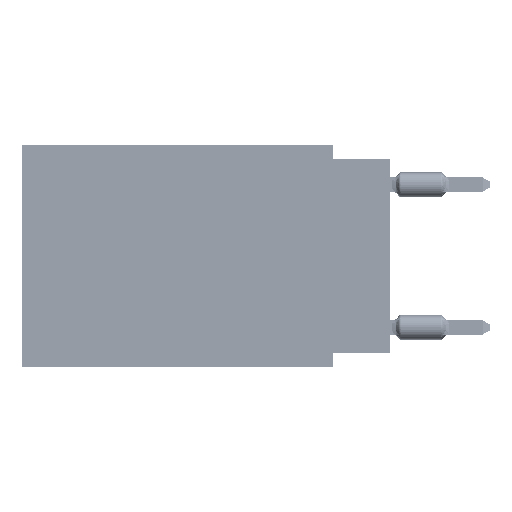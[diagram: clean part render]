
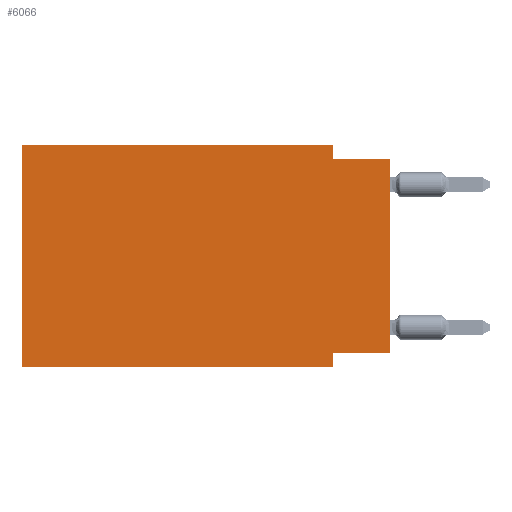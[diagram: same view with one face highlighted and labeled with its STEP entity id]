
A CAD part, left-side view. The second image highlights one B-rep face of the part: STEP entity #6066.
In plain terms, the highlighted planar face has unit normal (-1, 0, 0).
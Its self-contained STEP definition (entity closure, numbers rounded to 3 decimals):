
#112 = CARTESIAN_POINT ( 'NONE',  ( 0., 0., -0.635 ) ) ;
#335 = CARTESIAN_POINT ( 'NONE',  ( 0., 16.383, 0. ) ) ;
#832 = CARTESIAN_POINT ( 'NONE',  ( 0., 0., 0. ) ) ;
#1482 = VERTEX_POINT ( 'NONE', #50527 ) ;
#2255 = EDGE_CURVE ( 'NONE', #1482, #6139, #44850, .T. ) ;
#2520 = ORIENTED_EDGE ( 'NONE', *, *, #33516, .F. ) ;
#4196 = ORIENTED_EDGE ( 'NONE', *, *, #2255, .F. ) ;
#6066 = ADVANCED_FACE ( 'NONE', ( #63066 ), #68050, .F. ) ;
#6139 = VERTEX_POINT ( 'NONE', #7153 ) ;
#7153 = CARTESIAN_POINT ( 'NONE',  ( 0., 2.54, -9.271 ) ) ;
#11260 = LINE ( 'NONE', #35721, #62080 ) ;
#11363 = CARTESIAN_POINT ( 'NONE',  ( 0., 2.54, -9.906 ) ) ;
#12891 = VECTOR ( 'NONE', #19060, 1000. ) ;
#13397 = ORIENTED_EDGE ( 'NONE', *, *, #21280, .F. ) ;
#13488 = EDGE_CURVE ( 'NONE', #1482, #39501, #45140, .T. ) ;
#17955 = DIRECTION ( 'NONE',  ( 0., 0., -1. ) ) ;
#18657 = CARTESIAN_POINT ( 'NONE',  ( 0., 16.383, 0. ) ) ;
#19052 = ORIENTED_EDGE ( 'NONE', *, *, #48343, .F. ) ;
#19060 = DIRECTION ( 'NONE',  ( 0., 0., 1. ) ) ;
#20803 = DIRECTION ( 'NONE',  ( 0., -1., 0. ) ) ;
#21280 = EDGE_CURVE ( 'NONE', #30817, #39501, #76295, .T. ) ;
#23316 = ORIENTED_EDGE ( 'NONE', *, *, #63812, .T. ) ;
#26527 = DIRECTION ( 'NONE',  ( 0., 0., 1. ) ) ;
#29941 = DIRECTION ( 'NONE',  ( 0., -1., 0. ) ) ;
#30707 = EDGE_CURVE ( 'NONE', #58672, #34071, #48167, .T. ) ;
#30817 = VERTEX_POINT ( 'NONE', #61016 ) ;
#31261 = LINE ( 'NONE', #11363, #57601 ) ;
#31377 = DIRECTION ( 'NONE',  ( 0., 0., -1. ) ) ;
#31573 = CARTESIAN_POINT ( 'NONE',  ( 0., 16.383, -9.906 ) ) ;
#33516 = EDGE_CURVE ( 'NONE', #81199, #58672, #50927, .T. ) ;
#34071 = VERTEX_POINT ( 'NONE', #78583 ) ;
#34145 = CARTESIAN_POINT ( 'NONE',  ( 0., 16.383, 0. ) ) ;
#34903 = VECTOR ( 'NONE', #58479, 1000. ) ;
#35721 = CARTESIAN_POINT ( 'NONE',  ( 0., 16.383, -9.906 ) ) ;
#37008 = DIRECTION ( 'NONE',  ( 1., 0., 0. ) ) ;
#37573 = LINE ( 'NONE', #62820, #50398 ) ;
#38632 = CARTESIAN_POINT ( 'NONE',  ( 0., 0., -9.271 ) ) ;
#38904 = ORIENTED_EDGE ( 'NONE', *, *, #39510, .F. ) ;
#39501 = VERTEX_POINT ( 'NONE', #61196 ) ;
#39510 = EDGE_CURVE ( 'NONE', #34071, #30817, #37573, .T. ) ;
#44850 = LINE ( 'NONE', #38632, #34903 ) ;
#45140 = LINE ( 'NONE', #832, #55707 ) ;
#47963 = VECTOR ( 'NONE', #20803, 1000. ) ;
#48167 = LINE ( 'NONE', #34145, #56064 ) ;
#48343 = EDGE_CURVE ( 'NONE', #6139, #58126, #31261, .T. ) ;
#48999 = EDGE_LOOP ( 'NONE', ( #53182, #13397, #38904, #69527, #2520, #23316, #19052, #4196 ) ) ;
#49397 = CARTESIAN_POINT ( 'NONE',  ( 0., 16.383, 0. ) ) ;
#50398 = VECTOR ( 'NONE', #31377, 1000. ) ;
#50527 = CARTESIAN_POINT ( 'NONE',  ( 0., 0., -9.271 ) ) ;
#50927 = LINE ( 'NONE', #18657, #12891 ) ;
#53182 = ORIENTED_EDGE ( 'NONE', *, *, #13488, .T. ) ;
#55707 = VECTOR ( 'NONE', #26527, 1000. ) ;
#56064 = VECTOR ( 'NONE', #79227, 1000. ) ;
#56289 = AXIS2_PLACEMENT_3D ( 'NONE', #49397, #37008, #17955 ) ;
#57601 = VECTOR ( 'NONE', #61887, 1000. ) ;
#58126 = VERTEX_POINT ( 'NONE', #74149 ) ;
#58479 = DIRECTION ( 'NONE',  ( 0., 1., 0. ) ) ;
#58672 = VERTEX_POINT ( 'NONE', #335 ) ;
#61016 = CARTESIAN_POINT ( 'NONE',  ( 0., 2.54, -0.635 ) ) ;
#61196 = CARTESIAN_POINT ( 'NONE',  ( 0., 0., -0.635 ) ) ;
#61887 = DIRECTION ( 'NONE',  ( 0., 0., -1. ) ) ;
#62080 = VECTOR ( 'NONE', #29941, 1000. ) ;
#62820 = CARTESIAN_POINT ( 'NONE',  ( 0., 2.54, 0. ) ) ;
#63066 = FACE_OUTER_BOUND ( 'NONE', #48999, .T. ) ;
#63812 = EDGE_CURVE ( 'NONE', #81199, #58126, #11260, .T. ) ;
#68050 = PLANE ( 'NONE',  #56289 ) ;
#69527 = ORIENTED_EDGE ( 'NONE', *, *, #30707, .F. ) ;
#74149 = CARTESIAN_POINT ( 'NONE',  ( 0., 2.54, -9.906 ) ) ;
#76295 = LINE ( 'NONE', #112, #47963 ) ;
#78583 = CARTESIAN_POINT ( 'NONE',  ( 0., 2.54, 0. ) ) ;
#79227 = DIRECTION ( 'NONE',  ( 0., -1., 0. ) ) ;
#81199 = VERTEX_POINT ( 'NONE', #31573 ) ;
